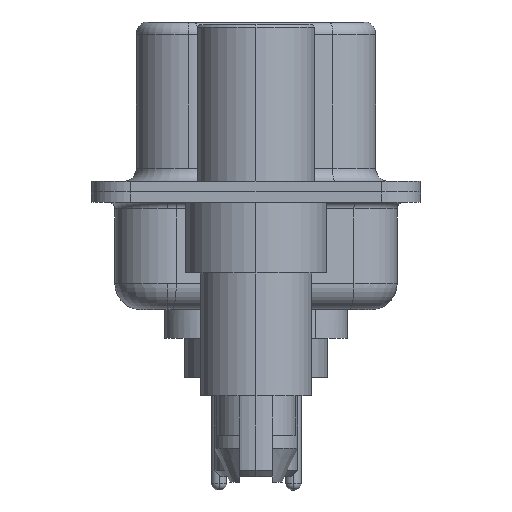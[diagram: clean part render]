
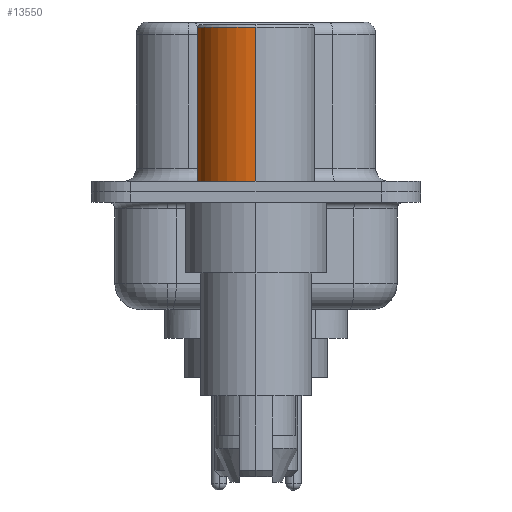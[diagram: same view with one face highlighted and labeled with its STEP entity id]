
A CAD part, left-side view. The second image highlights one B-rep face of the part: STEP entity #13550.
In plain terms, the highlighted cylindrical face has radius 2.25 mm (diameter 4.5 mm), a partial arc.
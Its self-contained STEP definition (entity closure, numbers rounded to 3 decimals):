
#1160 = DIRECTION ( 'NONE',  ( 1., 0., 0. ) ) ;
#1180 = VECTOR ( 'NONE', #9459, 1000. ) ;
#2801 = VERTEX_POINT ( 'NONE', #7068 ) ;
#3550 = DIRECTION ( 'NONE',  ( 1., 0., 0. ) ) ;
#4068 = AXIS2_PLACEMENT_3D ( 'NONE', #17232, #8027, #3550 ) ;
#4286 = VECTOR ( 'NONE', #17117, 1000. ) ;
#4514 = LINE ( 'NONE', #10907, #4286 ) ;
#5749 = VERTEX_POINT ( 'NONE', #8237 ) ;
#5966 = CIRCLE ( 'NONE', #10616, 2.25 ) ;
#6193 = EDGE_CURVE ( 'NONE', #7138, #2801, #12194, .T. ) ;
#6312 = AXIS2_PLACEMENT_3D ( 'NONE', #14676, #6948, #11479 ) ;
#6525 = ORIENTED_EDGE ( 'NONE', *, *, #19622, .F. ) ;
#6605 = EDGE_CURVE ( 'NONE', #5749, #2801, #5966, .T. ) ;
#6948 = DIRECTION ( 'NONE',  ( 0., 0., 1. ) ) ;
#7068 = CARTESIAN_POINT ( 'NONE',  ( -2.25, 0., 6.3 ) ) ;
#7138 = VERTEX_POINT ( 'NONE', #10044 ) ;
#8027 = DIRECTION ( 'NONE',  ( 0., 0., 1. ) ) ;
#8163 = CYLINDRICAL_SURFACE ( 'NONE', #4068, 2.25 ) ;
#8237 = CARTESIAN_POINT ( 'NONE',  ( 2.25, 0., 6.3 ) ) ;
#8512 = EDGE_CURVE ( 'NONE', #10632, #7138, #12596, .T. ) ;
#9459 = DIRECTION ( 'NONE',  ( 0., 0., 1. ) ) ;
#10044 = CARTESIAN_POINT ( 'NONE',  ( -2.25, 0., 0.4 ) ) ;
#10257 = DIRECTION ( 'NONE',  ( 0., 0., 1. ) ) ;
#10387 = CARTESIAN_POINT ( 'NONE',  ( 0., 0., 6.3 ) ) ;
#10616 = AXIS2_PLACEMENT_3D ( 'NONE', #10387, #10257, #1160 ) ;
#10632 = VERTEX_POINT ( 'NONE', #19109 ) ;
#10907 = CARTESIAN_POINT ( 'NONE',  ( 2.25, 0., 0.581 ) ) ;
#11292 = ORIENTED_EDGE ( 'NONE', *, *, #8512, .T. ) ;
#11479 = DIRECTION ( 'NONE',  ( 1., 0., 0. ) ) ;
#12194 = LINE ( 'NONE', #18617, #1180 ) ;
#12215 = FACE_OUTER_BOUND ( 'NONE', #15534, .T. ) ;
#12596 = CIRCLE ( 'NONE', #6312, 2.25 ) ;
#13550 = ADVANCED_FACE ( 'NONE', ( #12215 ), #8163, .T. ) ;
#14676 = CARTESIAN_POINT ( 'NONE',  ( 0., 0., 0.4 ) ) ;
#15534 = EDGE_LOOP ( 'NONE', ( #11292, #17074, #17438, #6525 ) ) ;
#17074 = ORIENTED_EDGE ( 'NONE', *, *, #6193, .T. ) ;
#17117 = DIRECTION ( 'NONE',  ( 0., 0., 1. ) ) ;
#17232 = CARTESIAN_POINT ( 'NONE',  ( 0., 0., 0.581 ) ) ;
#17438 = ORIENTED_EDGE ( 'NONE', *, *, #6605, .F. ) ;
#18617 = CARTESIAN_POINT ( 'NONE',  ( -2.25, 0., 0.581 ) ) ;
#19109 = CARTESIAN_POINT ( 'NONE',  ( 2.25, 0., 0.4 ) ) ;
#19622 = EDGE_CURVE ( 'NONE', #10632, #5749, #4514, .T. ) ;
